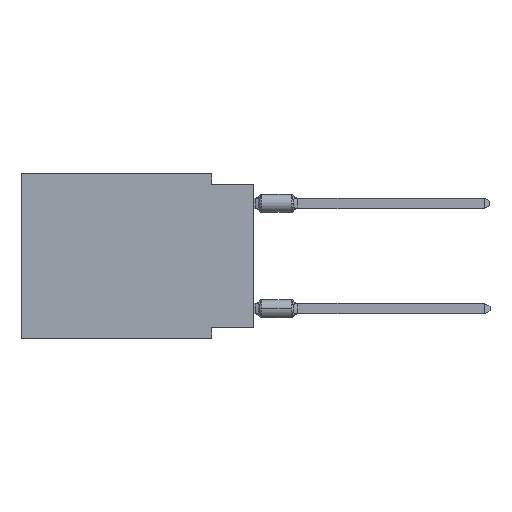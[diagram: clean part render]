
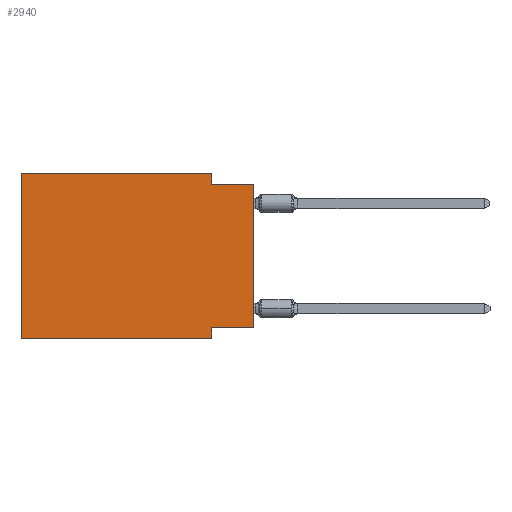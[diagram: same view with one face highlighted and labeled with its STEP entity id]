
A CAD part, left-side view. The second image highlights one B-rep face of the part: STEP entity #2940.
In plain terms, the highlighted planar face has unit normal (-1, 0, 0).
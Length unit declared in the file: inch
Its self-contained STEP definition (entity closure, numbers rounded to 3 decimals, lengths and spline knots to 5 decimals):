
#85 = LINE ( 'NONE', #5743, #3906 ) ;
#150 = EDGE_LOOP ( 'NONE', ( #1082, #13795, #15837, #13529, #611, #4725, #8376, #13364 ) ) ;
#494 = DIRECTION ( 'NONE',  ( 1., 0., 0. ) ) ;
#611 = ORIENTED_EDGE ( 'NONE', *, *, #815, .F. ) ;
#815 = EDGE_CURVE ( 'NONE', #8999, #1134, #10576, .T. ) ;
#853 = DIRECTION ( 'NONE',  ( 0., 0., -1. ) ) ;
#1082 = ORIENTED_EDGE ( 'NONE', *, *, #13976, .T. ) ;
#1088 = VERTEX_POINT ( 'NONE', #6985 ) ;
#1134 = VERTEX_POINT ( 'NONE', #9902 ) ;
#1250 = VECTOR ( 'NONE', #15300, 39.37008 ) ;
#1463 = CARTESIAN_POINT ( 'NONE',  ( 0., 0.1, -0.39 ) ) ;
#1608 = VECTOR ( 'NONE', #13943, 39.37008 ) ;
#1848 = EDGE_CURVE ( 'NONE', #8999, #5554, #85, .T. ) ;
#1897 = FACE_OUTER_BOUND ( 'NONE', #150, .T. ) ;
#2186 = EDGE_CURVE ( 'NONE', #1134, #11904, #6774, .T. ) ;
#2940 = ADVANCED_FACE ( 'NONE', ( #1897 ), #7660, .F. ) ;
#3255 = LINE ( 'NONE', #1463, #16544 ) ;
#3892 = CARTESIAN_POINT ( 'NONE',  ( 0., 0., -0.365 ) ) ;
#3906 = VECTOR ( 'NONE', #14565, 39.37008 ) ;
#4137 = VERTEX_POINT ( 'NONE', #11037 ) ;
#4249 = VECTOR ( 'NONE', #5231, 39.37008 ) ;
#4474 = DIRECTION ( 'NONE',  ( 0., 0., -1. ) ) ;
#4533 = DIRECTION ( 'NONE',  ( 0., 0., 1. ) ) ;
#4725 = ORIENTED_EDGE ( 'NONE', *, *, #1848, .T. ) ;
#5231 = DIRECTION ( 'NONE',  ( 0., 0., 1. ) ) ;
#5554 = VERTEX_POINT ( 'NONE', #6915 ) ;
#5725 = CARTESIAN_POINT ( 'NONE',  ( 0., 0.1, -0.365 ) ) ;
#5743 = CARTESIAN_POINT ( 'NONE',  ( 0., 0.55, -0.39 ) ) ;
#5950 = AXIS2_PLACEMENT_3D ( 'NONE', #13380, #494, #853 ) ;
#6581 = CARTESIAN_POINT ( 'NONE',  ( 0., 0.55, 0. ) ) ;
#6774 = LINE ( 'NONE', #6581, #1250 ) ;
#6915 = CARTESIAN_POINT ( 'NONE',  ( 0., 0.1, -0.39 ) ) ;
#6944 = EDGE_CURVE ( 'NONE', #1088, #4137, #10710, .T. ) ;
#6985 = CARTESIAN_POINT ( 'NONE',  ( 0., 0.1, -0.025 ) ) ;
#7270 = DIRECTION ( 'NONE',  ( 0., 0., -1. ) ) ;
#7458 = CARTESIAN_POINT ( 'NONE',  ( 0., 0.1, 0. ) ) ;
#7484 = VERTEX_POINT ( 'NONE', #3892 ) ;
#7660 = PLANE ( 'NONE',  #5950 ) ;
#7672 = CARTESIAN_POINT ( 'NONE',  ( 0., 0.55, 0. ) ) ;
#7910 = VECTOR ( 'NONE', #13703, 39.37008 ) ;
#8376 = ORIENTED_EDGE ( 'NONE', *, *, #13679, .F. ) ;
#8999 = VERTEX_POINT ( 'NONE', #9613 ) ;
#9399 = VECTOR ( 'NONE', #4533, 39.37008 ) ;
#9612 = LINE ( 'NONE', #10947, #1608 ) ;
#9613 = CARTESIAN_POINT ( 'NONE',  ( 0., 0.55, -0.39 ) ) ;
#9902 = CARTESIAN_POINT ( 'NONE',  ( 0., 0.55, 0. ) ) ;
#10184 = EDGE_CURVE ( 'NONE', #7484, #16540, #9612, .T. ) ;
#10576 = LINE ( 'NONE', #7672, #9399 ) ;
#10710 = LINE ( 'NONE', #17731, #7910 ) ;
#10947 = CARTESIAN_POINT ( 'NONE',  ( 0., 0., -0.365 ) ) ;
#11037 = CARTESIAN_POINT ( 'NONE',  ( 0., 0., -0.025 ) ) ;
#11214 = VECTOR ( 'NONE', #7270, 39.37008 ) ;
#11685 = LINE ( 'NONE', #7458, #11214 ) ;
#11904 = VERTEX_POINT ( 'NONE', #14021 ) ;
#13364 = ORIENTED_EDGE ( 'NONE', *, *, #10184, .F. ) ;
#13380 = CARTESIAN_POINT ( 'NONE',  ( 0., 0.55, 0. ) ) ;
#13529 = ORIENTED_EDGE ( 'NONE', *, *, #2186, .F. ) ;
#13679 = EDGE_CURVE ( 'NONE', #16540, #5554, #3255, .T. ) ;
#13703 = DIRECTION ( 'NONE',  ( 0., -1., 0. ) ) ;
#13795 = ORIENTED_EDGE ( 'NONE', *, *, #6944, .F. ) ;
#13943 = DIRECTION ( 'NONE',  ( 0., 1., 0. ) ) ;
#13976 = EDGE_CURVE ( 'NONE', #7484, #4137, #15640, .T. ) ;
#14021 = CARTESIAN_POINT ( 'NONE',  ( 0., 0.1, 0. ) ) ;
#14565 = DIRECTION ( 'NONE',  ( 0., -1., 0. ) ) ;
#15300 = DIRECTION ( 'NONE',  ( 0., -1., 0. ) ) ;
#15640 = LINE ( 'NONE', #18271, #4249 ) ;
#15723 = EDGE_CURVE ( 'NONE', #11904, #1088, #11685, .T. ) ;
#15837 = ORIENTED_EDGE ( 'NONE', *, *, #15723, .F. ) ;
#16540 = VERTEX_POINT ( 'NONE', #5725 ) ;
#16544 = VECTOR ( 'NONE', #4474, 39.37008 ) ;
#17731 = CARTESIAN_POINT ( 'NONE',  ( 0., 0., -0.025 ) ) ;
#18271 = CARTESIAN_POINT ( 'NONE',  ( 0., 0., 0. ) ) ;
